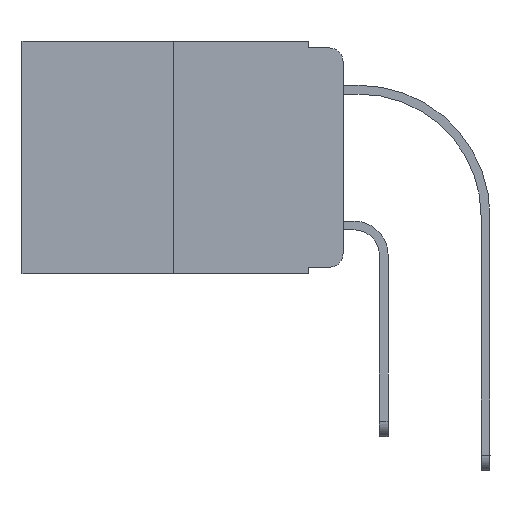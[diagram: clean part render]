
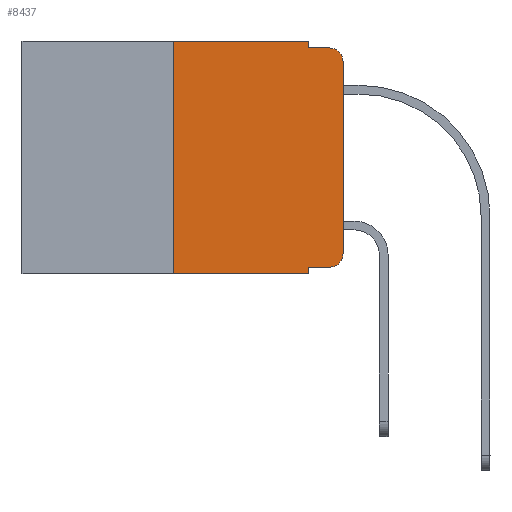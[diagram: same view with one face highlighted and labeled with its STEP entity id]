
A CAD part, left-side view. The second image highlights one B-rep face of the part: STEP entity #8437.
In plain terms, the highlighted planar face has unit normal (-1, 0, 0).
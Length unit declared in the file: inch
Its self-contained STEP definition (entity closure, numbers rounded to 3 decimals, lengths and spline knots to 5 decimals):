
#19 = CARTESIAN_POINT ( 'NONE',  ( 0., 0.051, -0.01 ) ) ;
#184 = CARTESIAN_POINT ( 'NONE',  ( 0., 0.051, 0. ) ) ;
#491 = VERTEX_POINT ( 'NONE', #7913 ) ;
#1021 = CARTESIAN_POINT ( 'NONE',  ( 0., 0.051, -0.01 ) ) ;
#1039 = CARTESIAN_POINT ( 'NONE',  ( 0., 0.02, -0.03 ) ) ;
#1043 = CARTESIAN_POINT ( 'NONE',  ( 0., 0., -0.03 ) ) ;
#1232 = LINE ( 'NONE', #11444, #15824 ) ;
#2252 = VECTOR ( 'NONE', #6292, 39.37008 ) ;
#2453 = DIRECTION ( 'NONE',  ( -1., 0., 0. ) ) ;
#2484 = EDGE_CURVE ( 'NONE', #12787, #5027, #10068, .T. ) ;
#2785 = EDGE_CURVE ( 'NONE', #4154, #18520, #17410, .T. ) ;
#4131 = DIRECTION ( 'NONE',  ( 0., 0., 1. ) ) ;
#4154 = VERTEX_POINT ( 'NONE', #1043 ) ;
#4413 = ORIENTED_EDGE ( 'NONE', *, *, #17828, .T. ) ;
#4524 = CARTESIAN_POINT ( 'NONE',  ( 0., 0.051, 0. ) ) ;
#5027 = VERTEX_POINT ( 'NONE', #16671 ) ;
#5049 = VERTEX_POINT ( 'NONE', #7764 ) ;
#5208 = ORIENTED_EDGE ( 'NONE', *, *, #7579, .T. ) ;
#5266 = LINE ( 'NONE', #16534, #9387 ) ;
#5314 = CARTESIAN_POINT ( 'NONE',  ( 0., 0.02, -0.313 ) ) ;
#5493 = PLANE ( 'NONE',  #17002 ) ;
#5693 = VERTEX_POINT ( 'NONE', #4524 ) ;
#5826 = AXIS2_PLACEMENT_3D ( 'NONE', #5314, #15452, #14142 ) ;
#5993 = DIRECTION ( 'NONE',  ( 0., 0., -1. ) ) ;
#6066 = EDGE_CURVE ( 'NONE', #11456, #18520, #11547, .T. ) ;
#6174 = LINE ( 'NONE', #184, #7666 ) ;
#6292 = DIRECTION ( 'NONE',  ( 0., 0., -1. ) ) ;
#6449 = EDGE_CURVE ( 'NONE', #5693, #11456, #6174, .T. ) ;
#6477 = VECTOR ( 'NONE', #9584, 39.37008 ) ;
#6656 = ORIENTED_EDGE ( 'NONE', *, *, #16354, .T. ) ;
#6752 = ORIENTED_EDGE ( 'NONE', *, *, #6066, .F. ) ;
#7577 = VECTOR ( 'NONE', #11009, 39.37008 ) ;
#7579 = EDGE_CURVE ( 'NONE', #5049, #4154, #1232, .T. ) ;
#7666 = VECTOR ( 'NONE', #5993, 39.37008 ) ;
#7764 = CARTESIAN_POINT ( 'NONE',  ( 0., 0., -0.313 ) ) ;
#7913 = CARTESIAN_POINT ( 'NONE',  ( 0., 0.051, -0.343 ) ) ;
#7971 = ORIENTED_EDGE ( 'NONE', *, *, #16751, .T. ) ;
#7983 = VERTEX_POINT ( 'NONE', #15366 ) ;
#8437 = ADVANCED_FACE ( 'NONE', ( #9717 ), #5493, .F. ) ;
#8941 = ORIENTED_EDGE ( 'NONE', *, *, #2484, .F. ) ;
#9066 = CARTESIAN_POINT ( 'NONE',  ( 0., 0.051, -0.333 ) ) ;
#9101 = CARTESIAN_POINT ( 'NONE',  ( 0., 0.051, 0. ) ) ;
#9320 = AXIS2_PLACEMENT_3D ( 'NONE', #1039, #2453, #16531 ) ;
#9387 = VECTOR ( 'NONE', #16441, 39.37008 ) ;
#9400 = CARTESIAN_POINT ( 'NONE',  ( 0., 0.25, -0.343 ) ) ;
#9584 = DIRECTION ( 'NONE',  ( 0., -1., 0. ) ) ;
#9608 = LINE ( 'NONE', #9066, #7577 ) ;
#9717 = FACE_OUTER_BOUND ( 'NONE', #17475, .T. ) ;
#9793 = CARTESIAN_POINT ( 'NONE',  ( 0., 0.25, 0. ) ) ;
#9817 = CARTESIAN_POINT ( 'NONE',  ( 0., 0.473, 0. ) ) ;
#10068 = LINE ( 'NONE', #9793, #16847 ) ;
#10491 = DIRECTION ( 'NONE',  ( 0., -1., 0. ) ) ;
#10703 = CARTESIAN_POINT ( 'NONE',  ( 0., 0.02, -0.01 ) ) ;
#11009 = DIRECTION ( 'NONE',  ( 0., -1., 0. ) ) ;
#11170 = LINE ( 'NONE', #15680, #6477 ) ;
#11444 = CARTESIAN_POINT ( 'NONE',  ( 0., 0., 0. ) ) ;
#11456 = VERTEX_POINT ( 'NONE', #1021 ) ;
#11547 = LINE ( 'NONE', #19, #12443 ) ;
#12443 = VECTOR ( 'NONE', #10491, 39.37008 ) ;
#12787 = VERTEX_POINT ( 'NONE', #9400 ) ;
#12887 = DIRECTION ( 'NONE',  ( 0., 0., 1. ) ) ;
#12932 = ORIENTED_EDGE ( 'NONE', *, *, #2785, .T. ) ;
#13016 = CARTESIAN_POINT ( 'NONE',  ( 0., 0.02, -0.333 ) ) ;
#13422 = LINE ( 'NONE', #9101, #2252 ) ;
#14136 = DIRECTION ( 'NONE',  ( 1., 0., 0. ) ) ;
#14142 = DIRECTION ( 'NONE',  ( 0., 0., -1. ) ) ;
#14301 = EDGE_CURVE ( 'NONE', #7983, #491, #13422, .T. ) ;
#14812 = CIRCLE ( 'NONE', #5826, 0.02 ) ;
#15341 = ORIENTED_EDGE ( 'NONE', *, *, #15631, .F. ) ;
#15366 = CARTESIAN_POINT ( 'NONE',  ( 0., 0.051, -0.333 ) ) ;
#15452 = DIRECTION ( 'NONE',  ( -1., 0., 0. ) ) ;
#15631 = EDGE_CURVE ( 'NONE', #5027, #5693, #11170, .T. ) ;
#15680 = CARTESIAN_POINT ( 'NONE',  ( 0., 0.473, 0. ) ) ;
#15824 = VECTOR ( 'NONE', #4131, 39.37008 ) ;
#16038 = ORIENTED_EDGE ( 'NONE', *, *, #6449, .F. ) ;
#16165 = VERTEX_POINT ( 'NONE', #13016 ) ;
#16354 = EDGE_CURVE ( 'NONE', #7983, #16165, #9608, .T. ) ;
#16441 = DIRECTION ( 'NONE',  ( 0., -1., 0. ) ) ;
#16531 = DIRECTION ( 'NONE',  ( 0., 0., -1. ) ) ;
#16534 = CARTESIAN_POINT ( 'NONE',  ( 0., 0.473, -0.343 ) ) ;
#16671 = CARTESIAN_POINT ( 'NONE',  ( 0., 0.25, 0. ) ) ;
#16751 = EDGE_CURVE ( 'NONE', #12787, #491, #5266, .T. ) ;
#16847 = VECTOR ( 'NONE', #12887, 39.37008 ) ;
#17002 = AXIS2_PLACEMENT_3D ( 'NONE', #9817, #14136, #18456 ) ;
#17410 = CIRCLE ( 'NONE', #9320, 0.02 ) ;
#17475 = EDGE_LOOP ( 'NONE', ( #5208, #12932, #6752, #16038, #15341, #8941, #7971, #18522, #6656, #4413 ) ) ;
#17828 = EDGE_CURVE ( 'NONE', #16165, #5049, #14812, .T. ) ;
#18456 = DIRECTION ( 'NONE',  ( 0., 0., -1. ) ) ;
#18520 = VERTEX_POINT ( 'NONE', #10703 ) ;
#18522 = ORIENTED_EDGE ( 'NONE', *, *, #14301, .F. ) ;
